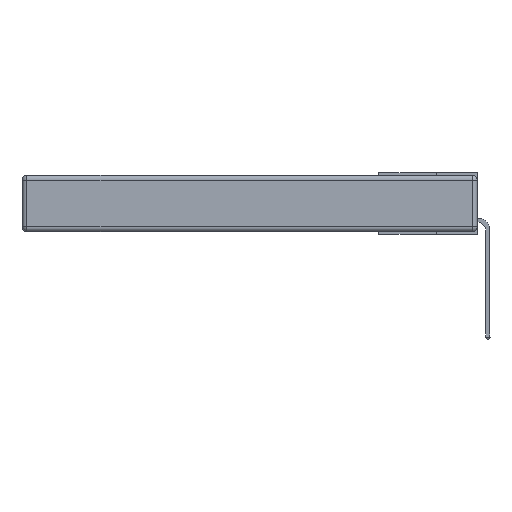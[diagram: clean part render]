
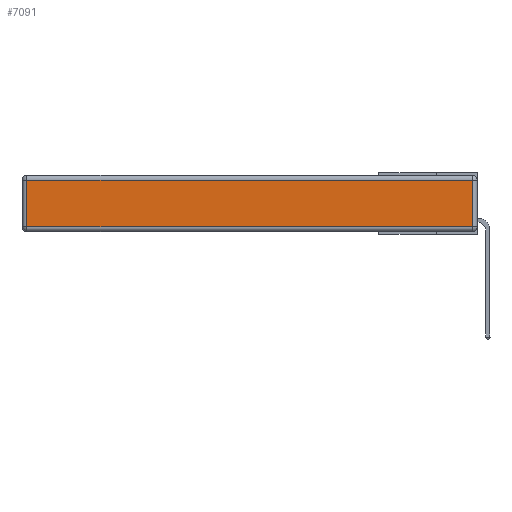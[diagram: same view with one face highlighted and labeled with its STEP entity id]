
A CAD part, left-side view. The second image highlights one B-rep face of the part: STEP entity #7091.
In plain terms, the highlighted planar face has unit normal (-1, 0, 0).
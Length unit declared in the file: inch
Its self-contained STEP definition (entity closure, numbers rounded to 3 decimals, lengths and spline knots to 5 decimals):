
#8 = CARTESIAN_POINT ( 'NONE',  ( 0., 2.75, -0.03 ) ) ;
#102 = DIRECTION ( 'NONE',  ( 0., 0., 1. ) ) ;
#254 = VERTEX_POINT ( 'NONE', #10200 ) ;
#757 = ORIENTED_EDGE ( 'NONE', *, *, #10042, .T. ) ;
#1349 = ORIENTED_EDGE ( 'NONE', *, *, #3937, .T. ) ;
#2951 = ORIENTED_EDGE ( 'NONE', *, *, #11643, .T. ) ;
#3071 = VECTOR ( 'NONE', #20084, 39.37008 ) ;
#3937 = EDGE_CURVE ( 'NONE', #254, #9010, #13435, .T. ) ;
#5137 = LINE ( 'NONE', #17978, #19182 ) ;
#5802 = CARTESIAN_POINT ( 'NONE',  ( 0., 0.03, -0.343 ) ) ;
#6690 = AXIS2_PLACEMENT_3D ( 'NONE', #17566, #17338, #102 ) ;
#7091 = ADVANCED_FACE ( 'NONE', ( #16206 ), #13713, .T. ) ;
#7891 = ORIENTED_EDGE ( 'NONE', *, *, #13567, .T. ) ;
#8259 = CARTESIAN_POINT ( 'NONE',  ( 0., 2.72, -0.03 ) ) ;
#8611 = DIRECTION ( 'NONE',  ( 0., 1., 0. ) ) ;
#9010 = VERTEX_POINT ( 'NONE', #19082 ) ;
#9641 = VECTOR ( 'NONE', #21617, 39.37008 ) ;
#10042 = EDGE_CURVE ( 'NONE', #20586, #254, #19013, .T. ) ;
#10200 = CARTESIAN_POINT ( 'NONE',  ( 0., 0.03, -0.313 ) ) ;
#10484 = VERTEX_POINT ( 'NONE', #8259 ) ;
#11643 = EDGE_CURVE ( 'NONE', #10484, #20586, #5137, .T. ) ;
#12831 = DIRECTION ( 'NONE',  ( 0., 0., -1. ) ) ;
#13435 = LINE ( 'NONE', #5802, #9641 ) ;
#13567 = EDGE_CURVE ( 'NONE', #9010, #10484, #16363, .T. ) ;
#13713 = PLANE ( 'NONE',  #6690 ) ;
#15536 = VECTOR ( 'NONE', #8611, 39.37008 ) ;
#16206 = FACE_OUTER_BOUND ( 'NONE', #19717, .T. ) ;
#16363 = LINE ( 'NONE', #8, #15536 ) ;
#16376 = CARTESIAN_POINT ( 'NONE',  ( 0., 0., -0.313 ) ) ;
#17186 = CARTESIAN_POINT ( 'NONE',  ( 0., 2.72, -0.313 ) ) ;
#17338 = DIRECTION ( 'NONE',  ( -1., 0., 0. ) ) ;
#17566 = CARTESIAN_POINT ( 'NONE',  ( 0., 0., -0.343 ) ) ;
#17978 = CARTESIAN_POINT ( 'NONE',  ( 0., 2.72, -0.343 ) ) ;
#19013 = LINE ( 'NONE', #16376, #3071 ) ;
#19082 = CARTESIAN_POINT ( 'NONE',  ( 0., 0.03, -0.03 ) ) ;
#19182 = VECTOR ( 'NONE', #12831, 39.37008 ) ;
#19717 = EDGE_LOOP ( 'NONE', ( #757, #1349, #7891, #2951 ) ) ;
#20084 = DIRECTION ( 'NONE',  ( 0., -1., 0. ) ) ;
#20586 = VERTEX_POINT ( 'NONE', #17186 ) ;
#21617 = DIRECTION ( 'NONE',  ( 0., 0., 1. ) ) ;
